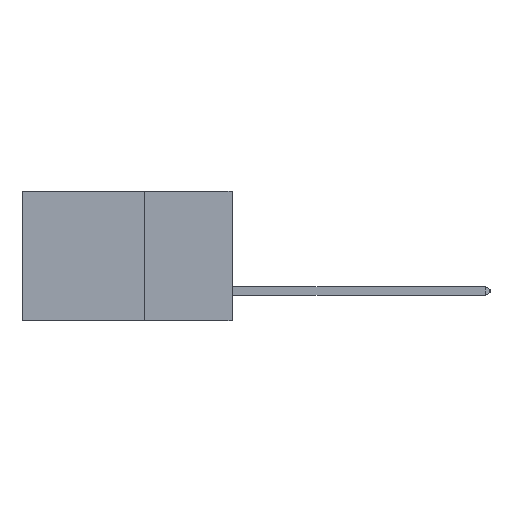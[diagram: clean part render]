
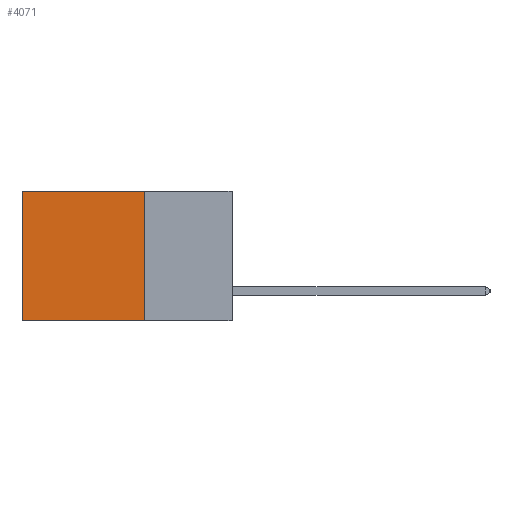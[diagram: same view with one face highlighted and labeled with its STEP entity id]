
A CAD part, left-side view. The second image highlights one B-rep face of the part: STEP entity #4071.
In plain terms, the highlighted planar face has unit normal (-1, 0, 0).
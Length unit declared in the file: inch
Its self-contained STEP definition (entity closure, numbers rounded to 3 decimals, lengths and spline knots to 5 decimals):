
#69 = CARTESIAN_POINT ( 'NONE',  ( 0.2875, 0.6, -0.37 ) ) ;
#187 = ORIENTED_EDGE ( 'NONE', *, *, #10538, .T. ) ;
#683 = DIRECTION ( 'NONE',  ( 0., 1., 0. ) ) ;
#1178 = VERTEX_POINT ( 'NONE', #8601 ) ;
#2886 = VERTEX_POINT ( 'NONE', #69 ) ;
#3267 = VERTEX_POINT ( 'NONE', #16890 ) ;
#4071 = ADVANCED_FACE ( 'NONE', ( #7573 ), #17460, .F. ) ;
#5008 = DIRECTION ( 'NONE',  ( 0., 1., 0. ) ) ;
#5119 = AXIS2_PLACEMENT_3D ( 'NONE', #15483, #23284, #5692 ) ;
#5249 = EDGE_LOOP ( 'NONE', ( #14839, #23497, #16097, #187 ) ) ;
#5692 = DIRECTION ( 'NONE',  ( 0., 0., -1. ) ) ;
#5812 = EDGE_CURVE ( 'NONE', #9417, #2886, #24136, .T. ) ;
#6261 = DIRECTION ( 'NONE',  ( 0., 0., -1. ) ) ;
#6523 = CARTESIAN_POINT ( 'NONE',  ( 0.2875, 0.25, -0.37 ) ) ;
#7485 = LINE ( 'NONE', #18032, #12694 ) ;
#7573 = FACE_OUTER_BOUND ( 'NONE', #5249, .T. ) ;
#8601 = CARTESIAN_POINT ( 'NONE',  ( 0.2875, 0.25, 0. ) ) ;
#9417 = VERTEX_POINT ( 'NONE', #13657 ) ;
#9427 = DIRECTION ( 'NONE',  ( 0., 0., -1. ) ) ;
#10538 = EDGE_CURVE ( 'NONE', #1178, #3267, #14060, .T. ) ;
#10901 = CARTESIAN_POINT ( 'NONE',  ( 0.2875, 0.25, 0. ) ) ;
#11509 = EDGE_CURVE ( 'NONE', #1178, #9417, #7485, .T. ) ;
#12694 = VECTOR ( 'NONE', #6261, 39.37008 ) ;
#13657 = CARTESIAN_POINT ( 'NONE',  ( 0.2875, 0.25, -0.37 ) ) ;
#14060 = LINE ( 'NONE', #10901, #24507 ) ;
#14839 = ORIENTED_EDGE ( 'NONE', *, *, #24995, .T. ) ;
#15483 = CARTESIAN_POINT ( 'NONE',  ( 0.2875, 0.25, 0. ) ) ;
#16097 = ORIENTED_EDGE ( 'NONE', *, *, #11509, .F. ) ;
#16890 = CARTESIAN_POINT ( 'NONE',  ( 0.2875, 0.6, 0. ) ) ;
#17460 = PLANE ( 'NONE',  #5119 ) ;
#18032 = CARTESIAN_POINT ( 'NONE',  ( 0.2875, 0.25, 0. ) ) ;
#21224 = CARTESIAN_POINT ( 'NONE',  ( 0.2875, 0.6, 0. ) ) ;
#21487 = LINE ( 'NONE', #21224, #23933 ) ;
#23284 = DIRECTION ( 'NONE',  ( 1., 0., 0. ) ) ;
#23497 = ORIENTED_EDGE ( 'NONE', *, *, #5812, .F. ) ;
#23521 = VECTOR ( 'NONE', #683, 39.37008 ) ;
#23933 = VECTOR ( 'NONE', #9427, 39.37008 ) ;
#24136 = LINE ( 'NONE', #6523, #23521 ) ;
#24507 = VECTOR ( 'NONE', #5008, 39.37008 ) ;
#24995 = EDGE_CURVE ( 'NONE', #3267, #2886, #21487, .T. ) ;
